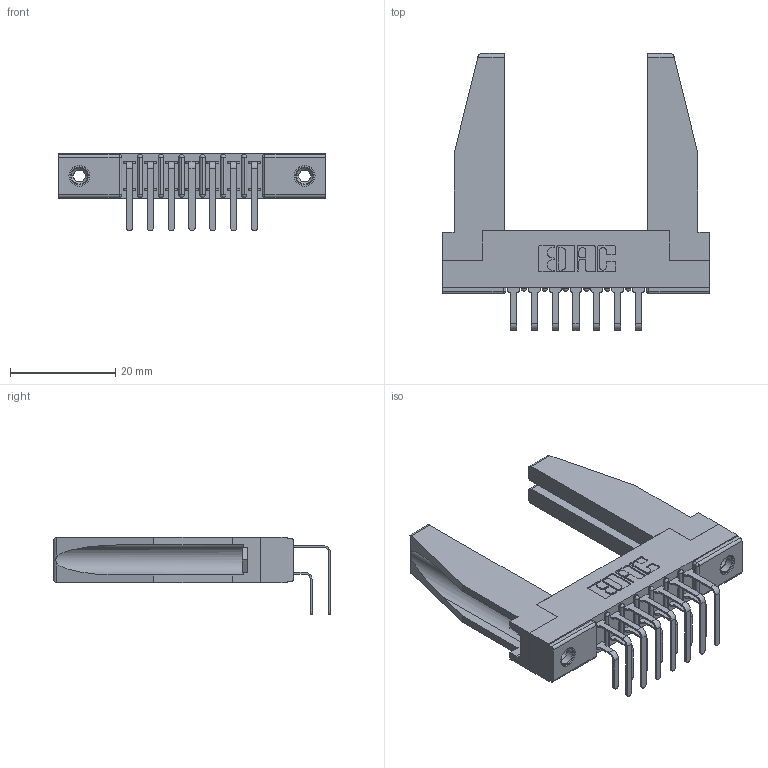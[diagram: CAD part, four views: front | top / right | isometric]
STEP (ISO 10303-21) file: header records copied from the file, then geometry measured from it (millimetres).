
FILE_DESCRIPTION (( 'STEP AP203' ), '1' );
FILE_NAME ('357-014-558-278.STEP', '2019-09-17T18:49:24', ( '' ), ( '' ), 'SwSTEP 2.0', 'SolidWorks 2016', '' );
FILE_SCHEMA (( 'CONFIG_CONTROL_DESIGN' ));
Length unit declared in the file: inch
Products named in the file (6): 345-250-001_345-250-001-102; 307-290-001_558 - 2 (Single); 307 Part_.156 Dia Mounting Holes; 357-014-558-278; 307-220-078; 307-290-001_558 559 - 1 (Single)
Assembly tree (19 placements, depth 2):
  357-014-558-278
    307 Part_.156 Dia Mounting Holes
    307-290-001_558 559 - 1 (Single)  x7
    307-290-001_558 - 2 (Single)  x7
    307-220-078  x2
    345-250-001_345-250-001-102  x2
Bounding box: 50.75 x 52.67 x 14.81 mm (x, y, z)
Volume: 7376.6 mm3; surface area: 9366.9 mm2
Topology: 19 solids, 19 shells, 956 faces, 2641 edges, 1710 vertices
Faces by surface type: plane 616, cylinder 308, sphere 16, cone 12, torus 4
Entity records: 14426 total; most frequent: CARTESIAN_POINT 2383, ORIENTED_EDGE 2316, DIRECTION 2302, EDGE_CURVE 1158, LINE 876, VECTOR 876, VERTEX_POINT 752, AXIS2_PLACEMENT_3D 713
